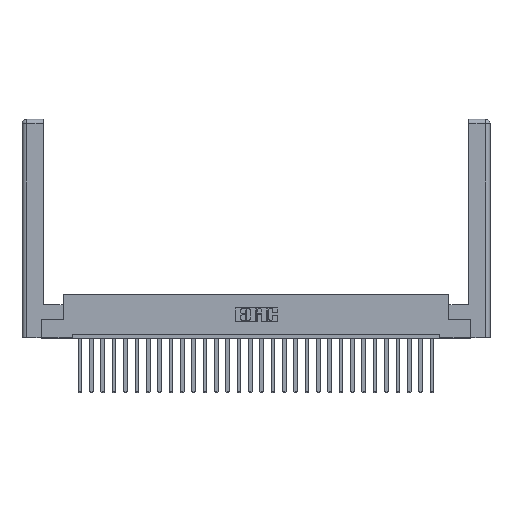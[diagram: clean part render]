
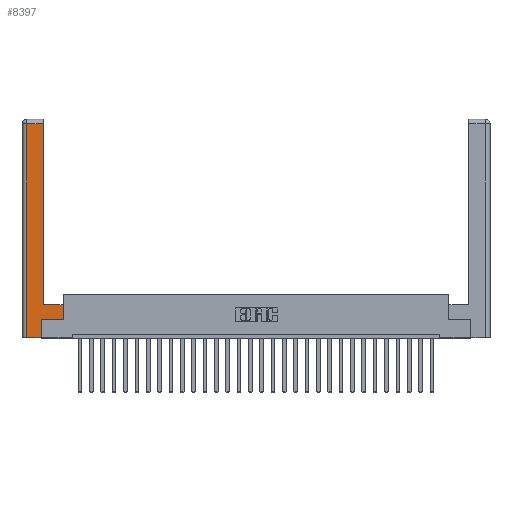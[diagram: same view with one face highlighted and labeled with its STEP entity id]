
A CAD part, top view. The second image highlights one B-rep face of the part: STEP entity #8397.
In plain terms, the highlighted planar face has unit normal (0, 0, 1).
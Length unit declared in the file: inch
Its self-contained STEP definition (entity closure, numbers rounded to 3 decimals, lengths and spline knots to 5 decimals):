
#165 = EDGE_CURVE ( 'NONE', #25706, #3542, #11449, .T. ) ;
#343 = VERTEX_POINT ( 'NONE', #7759 ) ;
#640 = DIRECTION ( 'NONE',  ( 0., 1., 0. ) ) ;
#841 = ORIENTED_EDGE ( 'NONE', *, *, #10577, .T. ) ;
#1213 = CARTESIAN_POINT ( 'NONE',  ( 0.295, 3., 0. ) ) ;
#1383 = CARTESIAN_POINT ( 'NONE',  ( 0.0615, 0., 0. ) ) ;
#2061 = VECTOR ( 'NONE', #10333, 39.37008 ) ;
#2690 = DIRECTION ( 'NONE',  ( 1., 0., 0. ) ) ;
#3488 = ORIENTED_EDGE ( 'NONE', *, *, #12398, .T. ) ;
#3542 = VERTEX_POINT ( 'NONE', #14831 ) ;
#4380 = DIRECTION ( 'NONE',  ( 0., 0., -1. ) ) ;
#4740 = LINE ( 'NONE', #18785, #2061 ) ;
#5065 = VERTEX_POINT ( 'NONE', #26392 ) ;
#5229 = VECTOR ( 'NONE', #7489, 39.37008 ) ;
#6473 = ORIENTED_EDGE ( 'NONE', *, *, #9968, .T. ) ;
#6883 = CARTESIAN_POINT ( 'NONE',  ( 0.265, 0.245, 0. ) ) ;
#7367 = CARTESIAN_POINT ( 'NONE',  ( 0.0615, 2.94, 0. ) ) ;
#7489 = DIRECTION ( 'NONE',  ( 0., 1., 0. ) ) ;
#7759 = CARTESIAN_POINT ( 'NONE',  ( 0.565, 0.245, 0. ) ) ;
#7957 = ORIENTED_EDGE ( 'NONE', *, *, #11442, .T. ) ;
#8071 = VECTOR ( 'NONE', #2690, 39.37008 ) ;
#8397 = ADVANCED_FACE ( 'NONE', ( #25997 ), #19379, .F. ) ;
#8669 = DIRECTION ( 'NONE',  ( -1., 0., 0. ) ) ;
#9968 = EDGE_CURVE ( 'NONE', #343, #23964, #22903, .T. ) ;
#10213 = CARTESIAN_POINT ( 'NONE',  ( 0.265, 0., 0. ) ) ;
#10333 = DIRECTION ( 'NONE',  ( -1., 0., 0. ) ) ;
#10577 = EDGE_CURVE ( 'NONE', #25317, #25706, #26858, .T. ) ;
#11442 = EDGE_CURVE ( 'NONE', #23964, #25317, #4740, .T. ) ;
#11449 = LINE ( 'NONE', #7367, #17119 ) ;
#11534 = DIRECTION ( 'NONE',  ( 0., 1., 0. ) ) ;
#12045 = LINE ( 'NONE', #16757, #20664 ) ;
#12176 = ORIENTED_EDGE ( 'NONE', *, *, #14712, .T. ) ;
#12398 = EDGE_CURVE ( 'NONE', #15096, #343, #12045, .T. ) ;
#12803 = CARTESIAN_POINT ( 'NONE',  ( 0., 0., 0. ) ) ;
#12967 = VECTOR ( 'NONE', #640, 39.37008 ) ;
#13592 = EDGE_LOOP ( 'NONE', ( #841, #19961, #16495, #22115, #12176, #3488, #6473, #7957 ) ) ;
#13740 = LINE ( 'NONE', #19971, #8071 ) ;
#13841 = CARTESIAN_POINT ( 'NONE',  ( 0.265, 0.245, 0. ) ) ;
#13867 = CARTESIAN_POINT ( 'NONE',  ( 0.565, 0.45, 0. ) ) ;
#13922 = DIRECTION ( 'NONE',  ( -1., 0., 0. ) ) ;
#14712 = EDGE_CURVE ( 'NONE', #17363, #15096, #20889, .T. ) ;
#14831 = CARTESIAN_POINT ( 'NONE',  ( 0.0615, 2.94, 0. ) ) ;
#15096 = VERTEX_POINT ( 'NONE', #13841 ) ;
#16495 = ORIENTED_EDGE ( 'NONE', *, *, #25835, .T. ) ;
#16665 = DIRECTION ( 'NONE',  ( 1., 0., 0. ) ) ;
#16757 = CARTESIAN_POINT ( 'NONE',  ( 0.565, 0.245, 0. ) ) ;
#17119 = VECTOR ( 'NONE', #13922, 39.37008 ) ;
#17363 = VERTEX_POINT ( 'NONE', #10213 ) ;
#18785 = CARTESIAN_POINT ( 'NONE',  ( 0.295, 0.45, 0. ) ) ;
#19379 = PLANE ( 'NONE',  #22146 ) ;
#19654 = CARTESIAN_POINT ( 'NONE',  ( 0.565, 0.45, 0. ) ) ;
#19875 = VECTOR ( 'NONE', #11534, 39.37008 ) ;
#19961 = ORIENTED_EDGE ( 'NONE', *, *, #165, .T. ) ;
#19971 = CARTESIAN_POINT ( 'NONE',  ( 0.265, 0., 0. ) ) ;
#20000 = CARTESIAN_POINT ( 'NONE',  ( 0.295, 2.94, 0. ) ) ;
#20378 = VECTOR ( 'NONE', #24751, 39.37008 ) ;
#20664 = VECTOR ( 'NONE', #16665, 39.37008 ) ;
#20889 = LINE ( 'NONE', #6883, #19875 ) ;
#21374 = LINE ( 'NONE', #1383, #20378 ) ;
#22115 = ORIENTED_EDGE ( 'NONE', *, *, #26313, .T. ) ;
#22146 = AXIS2_PLACEMENT_3D ( 'NONE', #12803, #4380, #8669 ) ;
#22497 = CARTESIAN_POINT ( 'NONE',  ( 0.295, 0.45, 0. ) ) ;
#22903 = LINE ( 'NONE', #19654, #12967 ) ;
#23964 = VERTEX_POINT ( 'NONE', #13867 ) ;
#24751 = DIRECTION ( 'NONE',  ( 0., -1., 0. ) ) ;
#25317 = VERTEX_POINT ( 'NONE', #22497 ) ;
#25706 = VERTEX_POINT ( 'NONE', #20000 ) ;
#25835 = EDGE_CURVE ( 'NONE', #3542, #5065, #21374, .T. ) ;
#25997 = FACE_OUTER_BOUND ( 'NONE', #13592, .T. ) ;
#26313 = EDGE_CURVE ( 'NONE', #5065, #17363, #13740, .T. ) ;
#26392 = CARTESIAN_POINT ( 'NONE',  ( 0.0615, 0., 0. ) ) ;
#26858 = LINE ( 'NONE', #1213, #5229 ) ;
